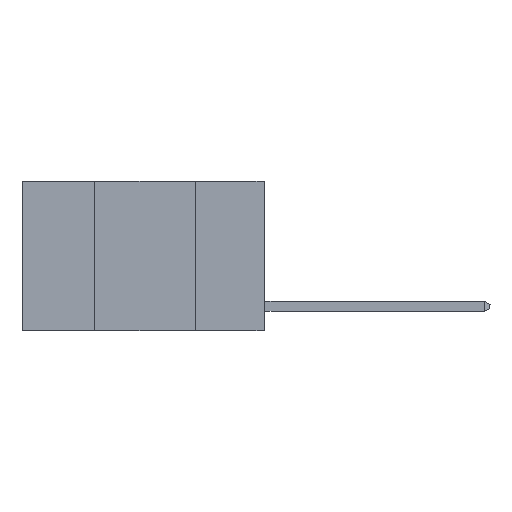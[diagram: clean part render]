
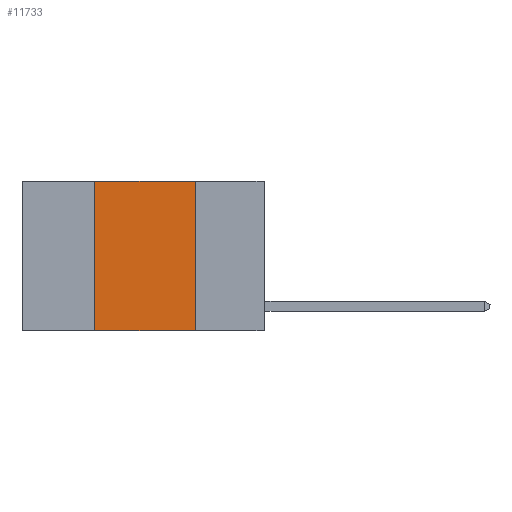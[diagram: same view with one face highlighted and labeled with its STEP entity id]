
A CAD part, left-side view. The second image highlights one B-rep face of the part: STEP entity #11733.
In plain terms, the highlighted planar face has unit normal (-1, 0, 0).
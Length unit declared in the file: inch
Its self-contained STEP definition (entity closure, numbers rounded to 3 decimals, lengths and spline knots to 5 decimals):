
#1456 = EDGE_CURVE ( 'NONE', #2455, #4497, #8774, .T. ) ;
#2455 = VERTEX_POINT ( 'NONE', #12852 ) ;
#2786 = VERTEX_POINT ( 'NONE', #16473 ) ;
#2832 = EDGE_CURVE ( 'NONE', #2786, #11727, #12110, .T. ) ;
#3076 = CARTESIAN_POINT ( 'NONE',  ( 0., 0.17, 0. ) ) ;
#3173 = CARTESIAN_POINT ( 'NONE',  ( 0., 0.6, 0. ) ) ;
#3832 = VECTOR ( 'NONE', #16492, 39.37008 ) ;
#4497 = VERTEX_POINT ( 'NONE', #14143 ) ;
#4500 = VECTOR ( 'NONE', #7797, 39.37008 ) ;
#4656 = CARTESIAN_POINT ( 'NONE',  ( 0., 0.42, 0. ) ) ;
#5152 = EDGE_LOOP ( 'NONE', ( #6828, #11837, #10341, #16182 ) ) ;
#6574 = CARTESIAN_POINT ( 'NONE',  ( 0., 0.6, 0. ) ) ;
#6828 = ORIENTED_EDGE ( 'NONE', *, *, #1456, .F. ) ;
#7797 = DIRECTION ( 'NONE',  ( 0., -1., 0. ) ) ;
#8049 = AXIS2_PLACEMENT_3D ( 'NONE', #3173, #12698, #11528 ) ;
#8178 = EDGE_CURVE ( 'NONE', #2786, #4497, #15888, .T. ) ;
#8492 = VECTOR ( 'NONE', #8702, 39.37008 ) ;
#8702 = DIRECTION ( 'NONE',  ( 0., 0., 1. ) ) ;
#8774 = LINE ( 'NONE', #3076, #3832 ) ;
#9221 = LINE ( 'NONE', #6574, #4500 ) ;
#9707 = VECTOR ( 'NONE', #14277, 39.37008 ) ;
#9714 = EDGE_CURVE ( 'NONE', #11727, #2455, #9221, .T. ) ;
#9830 = CARTESIAN_POINT ( 'NONE',  ( 0., 0.42, 0. ) ) ;
#10041 = CARTESIAN_POINT ( 'NONE',  ( 0., 0.6, -0.37 ) ) ;
#10341 = ORIENTED_EDGE ( 'NONE', *, *, #2832, .F. ) ;
#11528 = DIRECTION ( 'NONE',  ( 0., 0., -1. ) ) ;
#11727 = VERTEX_POINT ( 'NONE', #4656 ) ;
#11733 = ADVANCED_FACE ( 'NONE', ( #16002 ), #15445, .F. ) ;
#11837 = ORIENTED_EDGE ( 'NONE', *, *, #9714, .F. ) ;
#12110 = LINE ( 'NONE', #9830, #8492 ) ;
#12698 = DIRECTION ( 'NONE',  ( 1., 0., 0. ) ) ;
#12852 = CARTESIAN_POINT ( 'NONE',  ( 0., 0.17, 0. ) ) ;
#14143 = CARTESIAN_POINT ( 'NONE',  ( 0., 0.17, -0.37 ) ) ;
#14277 = DIRECTION ( 'NONE',  ( 0., -1., 0. ) ) ;
#15445 = PLANE ( 'NONE',  #8049 ) ;
#15888 = LINE ( 'NONE', #10041, #9707 ) ;
#16002 = FACE_OUTER_BOUND ( 'NONE', #5152, .T. ) ;
#16182 = ORIENTED_EDGE ( 'NONE', *, *, #8178, .T. ) ;
#16473 = CARTESIAN_POINT ( 'NONE',  ( 0., 0.42, -0.37 ) ) ;
#16492 = DIRECTION ( 'NONE',  ( 0., 0., -1. ) ) ;
